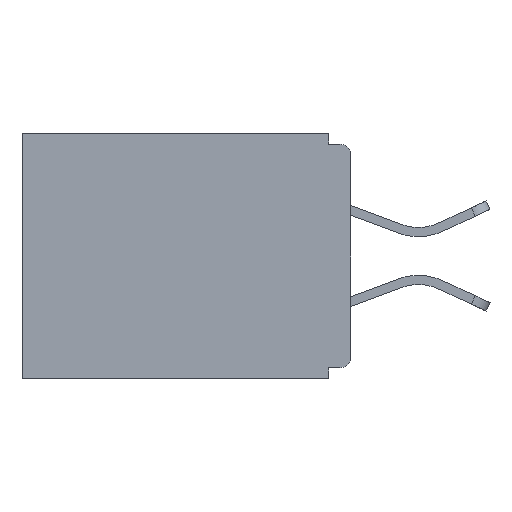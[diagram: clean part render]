
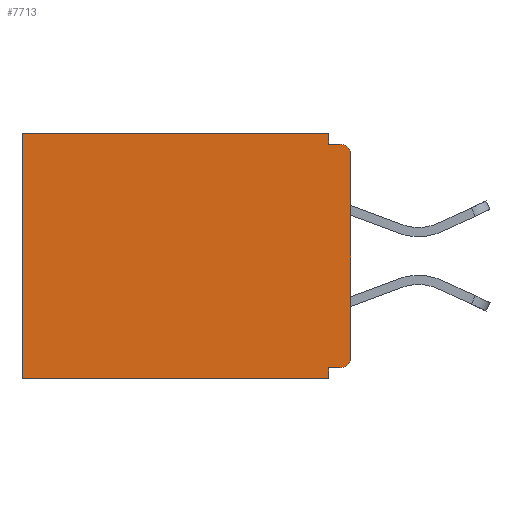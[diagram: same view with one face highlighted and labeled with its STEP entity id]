
A CAD part, left-side view. The second image highlights one B-rep face of the part: STEP entity #7713.
In plain terms, the highlighted planar face has unit normal (-1, 0, 0).
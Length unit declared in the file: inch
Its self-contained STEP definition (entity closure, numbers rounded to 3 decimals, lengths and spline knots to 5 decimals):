
#296 = VERTEX_POINT ( 'NONE', #12859 ) ;
#421 = EDGE_CURVE ( 'NONE', #6911, #296, #4621, .T. ) ;
#524 = EDGE_CURVE ( 'NONE', #966, #6911, #2402, .T. ) ;
#555 = ORIENTED_EDGE ( 'NONE', *, *, #13821, .F. ) ;
#699 = EDGE_CURVE ( 'NONE', #966, #12798, #8715, .T. ) ;
#966 = VERTEX_POINT ( 'NONE', #4079 ) ;
#1001 = DIRECTION ( 'NONE',  ( 0., 0., -1. ) ) ;
#1177 = VERTEX_POINT ( 'NONE', #4467 ) ;
#1211 = ORIENTED_EDGE ( 'NONE', *, *, #699, .T. ) ;
#1708 = ORIENTED_EDGE ( 'NONE', *, *, #10757, .F. ) ;
#2402 = LINE ( 'NONE', #11214, #8962 ) ;
#2503 = LINE ( 'NONE', #17585, #19420 ) ;
#2670 = DIRECTION ( 'NONE',  ( -1., 0., 0. ) ) ;
#2867 = VECTOR ( 'NONE', #1001, 39.37008 ) ;
#3052 = FACE_OUTER_BOUND ( 'NONE', #11659, .T. ) ;
#3688 = ORIENTED_EDGE ( 'NONE', *, *, #18986, .T. ) ;
#4079 = CARTESIAN_POINT ( 'NONE',  ( 0.298, 0.031, 0. ) ) ;
#4321 = EDGE_CURVE ( 'NONE', #16909, #296, #19168, .T. ) ;
#4467 = CARTESIAN_POINT ( 'NONE',  ( 0.298, 0., -0.313 ) ) ;
#4621 = LINE ( 'NONE', #5767, #9564 ) ;
#5134 = DIRECTION ( 'NONE',  ( 0., 1., 0. ) ) ;
#5141 = CARTESIAN_POINT ( 'NONE',  ( 0.298, 0., 0. ) ) ;
#5327 = DIRECTION ( 'NONE',  ( 0., 1., 0. ) ) ;
#5437 = ORIENTED_EDGE ( 'NONE', *, *, #524, .F. ) ;
#5625 = CARTESIAN_POINT ( 'NONE',  ( 0.298, 0.031, -0.015 ) ) ;
#5632 = ORIENTED_EDGE ( 'NONE', *, *, #5804, .F. ) ;
#5740 = ORIENTED_EDGE ( 'NONE', *, *, #421, .F. ) ;
#5767 = CARTESIAN_POINT ( 'NONE',  ( 0.298, 0., -0.015 ) ) ;
#5804 = EDGE_CURVE ( 'NONE', #19441, #7445, #18452, .T. ) ;
#5891 = DIRECTION ( 'NONE',  ( -1., 0., 0. ) ) ;
#6323 = EDGE_CURVE ( 'NONE', #12942, #1177, #11097, .T. ) ;
#6697 = VECTOR ( 'NONE', #18721, 39.37008 ) ;
#6911 = VERTEX_POINT ( 'NONE', #5625 ) ;
#7208 = CARTESIAN_POINT ( 'NONE',  ( 0.298, 0.031, -0.328 ) ) ;
#7347 = CARTESIAN_POINT ( 'NONE',  ( 0.298, 0.015, -0.313 ) ) ;
#7445 = VERTEX_POINT ( 'NONE', #11222 ) ;
#7468 = CARTESIAN_POINT ( 'NONE',  ( 0.298, 0.46, -0.343 ) ) ;
#7543 = VECTOR ( 'NONE', #5134, 39.37008 ) ;
#7713 = ADVANCED_FACE ( 'NONE', ( #3052 ), #10991, .F. ) ;
#8224 = CARTESIAN_POINT ( 'NONE',  ( 0.298, 0., -0.328 ) ) ;
#8715 = LINE ( 'NONE', #9611, #7543 ) ;
#8764 = AXIS2_PLACEMENT_3D ( 'NONE', #7347, #5891, #16676 ) ;
#8951 = VECTOR ( 'NONE', #5327, 39.37008 ) ;
#8962 = VECTOR ( 'NONE', #18912, 39.37008 ) ;
#9564 = VECTOR ( 'NONE', #17672, 39.37008 ) ;
#9611 = CARTESIAN_POINT ( 'NONE',  ( 0.298, 0., 0. ) ) ;
#10711 = VERTEX_POINT ( 'NONE', #7468 ) ;
#10757 = EDGE_CURVE ( 'NONE', #7445, #10711, #17317, .T. ) ;
#10991 = PLANE ( 'NONE',  #14692 ) ;
#11097 = CIRCLE ( 'NONE', #8764, 0.015 ) ;
#11214 = CARTESIAN_POINT ( 'NONE',  ( 0.298, 0.031, -0.343 ) ) ;
#11222 = CARTESIAN_POINT ( 'NONE',  ( 0.298, 0.031, -0.343 ) ) ;
#11380 = CARTESIAN_POINT ( 'NONE',  ( 0.298, 0.031, -0.343 ) ) ;
#11474 = CARTESIAN_POINT ( 'NONE',  ( 0.298, 0.015, -0.03 ) ) ;
#11659 = EDGE_LOOP ( 'NONE', ( #15653, #5740, #5437, #1211, #3688, #1708, #5632, #13825, #16339, #555 ) ) ;
#11783 = DIRECTION ( 'NONE',  ( 0., 0., -1. ) ) ;
#12457 = DIRECTION ( 'NONE',  ( 1., 0., 0. ) ) ;
#12798 = VERTEX_POINT ( 'NONE', #14464 ) ;
#12859 = CARTESIAN_POINT ( 'NONE',  ( 0.298, 0.015, -0.015 ) ) ;
#12942 = VERTEX_POINT ( 'NONE', #17724 ) ;
#13069 = DIRECTION ( 'NONE',  ( 0., 0., -1. ) ) ;
#13172 = DIRECTION ( 'NONE',  ( 0., 0., -1. ) ) ;
#13301 = CARTESIAN_POINT ( 'NONE',  ( 0.298, 0., -0.03 ) ) ;
#13821 = EDGE_CURVE ( 'NONE', #16909, #1177, #2503, .T. ) ;
#13825 = ORIENTED_EDGE ( 'NONE', *, *, #17184, .F. ) ;
#14115 = LINE ( 'NONE', #8224, #8951 ) ;
#14342 = CARTESIAN_POINT ( 'NONE',  ( 0.298, 0., -0.343 ) ) ;
#14464 = CARTESIAN_POINT ( 'NONE',  ( 0.298, 0.46, 0. ) ) ;
#14692 = AXIS2_PLACEMENT_3D ( 'NONE', #5141, #12457, #15635 ) ;
#15480 = VECTOR ( 'NONE', #11783, 39.37008 ) ;
#15635 = DIRECTION ( 'NONE',  ( 0., 0., -1. ) ) ;
#15653 = ORIENTED_EDGE ( 'NONE', *, *, #4321, .T. ) ;
#16339 = ORIENTED_EDGE ( 'NONE', *, *, #6323, .T. ) ;
#16676 = DIRECTION ( 'NONE',  ( 0., 0., -1. ) ) ;
#16909 = VERTEX_POINT ( 'NONE', #13301 ) ;
#17184 = EDGE_CURVE ( 'NONE', #12942, #19441, #14115, .T. ) ;
#17317 = LINE ( 'NONE', #14342, #6697 ) ;
#17585 = CARTESIAN_POINT ( 'NONE',  ( 0.298, 0., 0. ) ) ;
#17593 = AXIS2_PLACEMENT_3D ( 'NONE', #11474, #2670, #13172 ) ;
#17672 = DIRECTION ( 'NONE',  ( 0., -1., 0. ) ) ;
#17701 = CARTESIAN_POINT ( 'NONE',  ( 0.298, 0.46, 0. ) ) ;
#17724 = CARTESIAN_POINT ( 'NONE',  ( 0.298, 0.015, -0.328 ) ) ;
#18452 = LINE ( 'NONE', #11380, #2867 ) ;
#18721 = DIRECTION ( 'NONE',  ( 0., 1., 0. ) ) ;
#18795 = LINE ( 'NONE', #17701, #15480 ) ;
#18912 = DIRECTION ( 'NONE',  ( 0., 0., -1. ) ) ;
#18986 = EDGE_CURVE ( 'NONE', #12798, #10711, #18795, .T. ) ;
#19168 = CIRCLE ( 'NONE', #17593, 0.015 ) ;
#19420 = VECTOR ( 'NONE', #13069, 39.37008 ) ;
#19441 = VERTEX_POINT ( 'NONE', #7208 ) ;
